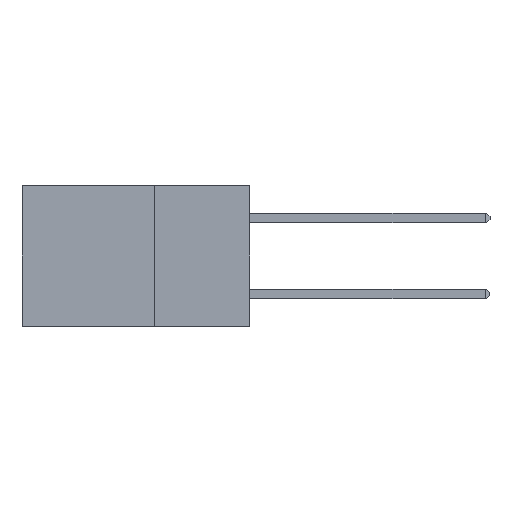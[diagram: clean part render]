
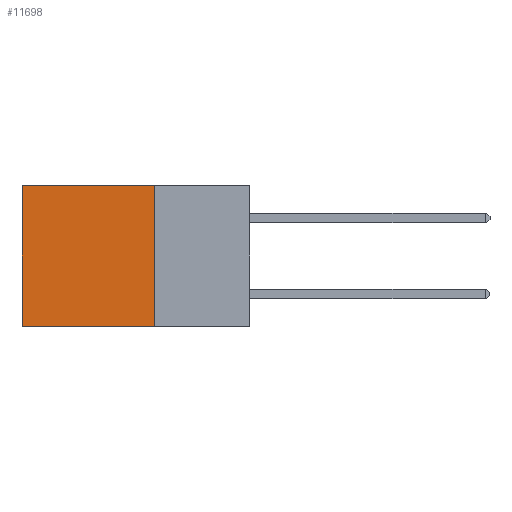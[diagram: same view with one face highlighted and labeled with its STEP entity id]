
A CAD part, left-side view. The second image highlights one B-rep face of the part: STEP entity #11698.
In plain terms, the highlighted planar face has unit normal (-1, 0, 0).
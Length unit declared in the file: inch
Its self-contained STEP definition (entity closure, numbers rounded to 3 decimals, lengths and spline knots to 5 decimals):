
#53 = LINE ( 'NONE', #7274, #8538 ) ;
#175 = CARTESIAN_POINT ( 'NONE',  ( 0.2875, 0.25, 0. ) ) ;
#190 = CARTESIAN_POINT ( 'NONE',  ( 0.2875, 0.6, -0.37 ) ) ;
#924 = DIRECTION ( 'NONE',  ( 0., 0., -1. ) ) ;
#1009 = EDGE_LOOP ( 'NONE', ( #15497, #5945, #4306, #5823 ) ) ;
#1367 = VECTOR ( 'NONE', #5145, 39.37008 ) ;
#1485 = CARTESIAN_POINT ( 'NONE',  ( 0.2875, 0.6, 0. ) ) ;
#2101 = VERTEX_POINT ( 'NONE', #190 ) ;
#2185 = EDGE_CURVE ( 'NONE', #14447, #2101, #53, .T. ) ;
#3080 = PLANE ( 'NONE',  #19489 ) ;
#4306 = ORIENTED_EDGE ( 'NONE', *, *, #5956, .F. ) ;
#4807 = DIRECTION ( 'NONE',  ( 0., 0., -1. ) ) ;
#4951 = LINE ( 'NONE', #14172, #17312 ) ;
#5145 = DIRECTION ( 'NONE',  ( 0., 0., -1. ) ) ;
#5823 = ORIENTED_EDGE ( 'NONE', *, *, #6530, .T. ) ;
#5945 = ORIENTED_EDGE ( 'NONE', *, *, #2185, .F. ) ;
#5956 = EDGE_CURVE ( 'NONE', #21111, #14447, #4951, .T. ) ;
#6530 = EDGE_CURVE ( 'NONE', #21111, #11763, #20032, .T. ) ;
#7274 = CARTESIAN_POINT ( 'NONE',  ( 0.2875, 0.25, -0.37 ) ) ;
#8025 = CARTESIAN_POINT ( 'NONE',  ( 0.2875, 0.25, 0. ) ) ;
#8538 = VECTOR ( 'NONE', #18493, 39.37008 ) ;
#10947 = DIRECTION ( 'NONE',  ( 0., 1., 0. ) ) ;
#11698 = ADVANCED_FACE ( 'NONE', ( #13101 ), #3080, .F. ) ;
#11763 = VERTEX_POINT ( 'NONE', #1485 ) ;
#13101 = FACE_OUTER_BOUND ( 'NONE', #1009, .T. ) ;
#13220 = CARTESIAN_POINT ( 'NONE',  ( 0.2875, 0.6, 0. ) ) ;
#14172 = CARTESIAN_POINT ( 'NONE',  ( 0.2875, 0.25, 0. ) ) ;
#14447 = VERTEX_POINT ( 'NONE', #16757 ) ;
#14526 = LINE ( 'NONE', #13220, #1367 ) ;
#14538 = DIRECTION ( 'NONE',  ( 1., 0., 0. ) ) ;
#15497 = ORIENTED_EDGE ( 'NONE', *, *, #15752, .T. ) ;
#15752 = EDGE_CURVE ( 'NONE', #11763, #2101, #14526, .T. ) ;
#15797 = CARTESIAN_POINT ( 'NONE',  ( 0.2875, 0.25, 0. ) ) ;
#16757 = CARTESIAN_POINT ( 'NONE',  ( 0.2875, 0.25, -0.37 ) ) ;
#17312 = VECTOR ( 'NONE', #924, 39.37008 ) ;
#18493 = DIRECTION ( 'NONE',  ( 0., 1., 0. ) ) ;
#19026 = VECTOR ( 'NONE', #10947, 39.37008 ) ;
#19489 = AXIS2_PLACEMENT_3D ( 'NONE', #8025, #14538, #4807 ) ;
#20032 = LINE ( 'NONE', #15797, #19026 ) ;
#21111 = VERTEX_POINT ( 'NONE', #175 ) ;
